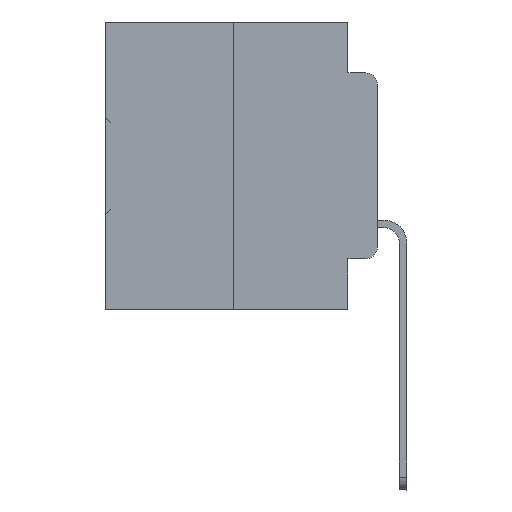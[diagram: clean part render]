
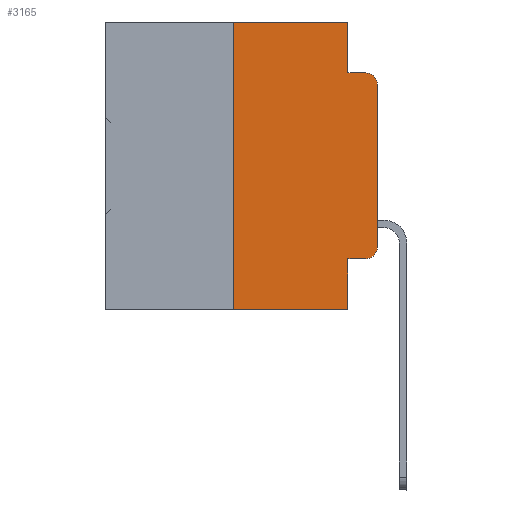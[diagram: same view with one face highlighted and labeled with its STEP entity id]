
A CAD part, left-side view. The second image highlights one B-rep face of the part: STEP entity #3165.
In plain terms, the highlighted planar face has unit normal (-1, 0, 0).
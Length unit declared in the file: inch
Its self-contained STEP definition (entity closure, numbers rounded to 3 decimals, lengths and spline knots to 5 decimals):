
#842 = VERTEX_POINT ( 'NONE', #8794 ) ;
#2227 = CARTESIAN_POINT ( 'NONE',  ( 0., 0.473, 0. ) ) ;
#2470 = EDGE_CURVE ( 'NONE', #12422, #8862, #34350, .T. ) ;
#3095 = DIRECTION ( 'NONE',  ( 0., 0., -1. ) ) ;
#3165 = ADVANCED_FACE ( 'NONE', ( #5425 ), #16175, .F. ) ;
#3203 = EDGE_CURVE ( 'NONE', #30793, #17209, #19401, .T. ) ;
#3281 = DIRECTION ( 'NONE',  ( 0., -1., 0. ) ) ;
#3731 = DIRECTION ( 'NONE',  ( 0., 0., 1. ) ) ;
#3785 = EDGE_CURVE ( 'NONE', #31473, #30793, #11796, .T. ) ;
#5024 = EDGE_CURVE ( 'NONE', #34529, #12422, #36636, .T. ) ;
#5371 = DIRECTION ( 'NONE',  ( 0., -1., 0. ) ) ;
#5425 = FACE_OUTER_BOUND ( 'NONE', #35494, .T. ) ;
#6071 = CARTESIAN_POINT ( 'NONE',  ( 0., 0.051, -0.4115 ) ) ;
#6695 = CARTESIAN_POINT ( 'NONE',  ( 0., 0.02, -0.4115 ) ) ;
#6772 = VERTEX_POINT ( 'NONE', #8458 ) ;
#7511 = DIRECTION ( 'NONE',  ( 0., 0., -1. ) ) ;
#7954 = CARTESIAN_POINT ( 'NONE',  ( 0., 0.051, -0.4115 ) ) ;
#8458 = CARTESIAN_POINT ( 'NONE',  ( 0., 0., -0.1085 ) ) ;
#8794 = CARTESIAN_POINT ( 'NONE',  ( 0., 0.051, -0.0885 ) ) ;
#8862 = VERTEX_POINT ( 'NONE', #14887 ) ;
#9082 = DIRECTION ( 'NONE',  ( -1., 0., 0. ) ) ;
#9260 = LINE ( 'NONE', #12468, #31121 ) ;
#9449 = DIRECTION ( 'NONE',  ( 0., 0., -1. ) ) ;
#11107 = DIRECTION ( 'NONE',  ( 1., 0., 0. ) ) ;
#11164 = VECTOR ( 'NONE', #29727, 39.37008 ) ;
#11585 = CARTESIAN_POINT ( 'NONE',  ( 0., 0.473, -0.5 ) ) ;
#11796 = LINE ( 'NONE', #25756, #29286 ) ;
#12168 = VECTOR ( 'NONE', #5371, 39.37008 ) ;
#12422 = VERTEX_POINT ( 'NONE', #6695 ) ;
#12468 = CARTESIAN_POINT ( 'NONE',  ( 0., 0.051, 0. ) ) ;
#12477 = DIRECTION ( 'NONE',  ( 0., 0., -1. ) ) ;
#12988 = ORIENTED_EDGE ( 'NONE', *, *, #3203, .F. ) ;
#13406 = ORIENTED_EDGE ( 'NONE', *, *, #15177, .T. ) ;
#14860 = LINE ( 'NONE', #18077, #25777 ) ;
#14887 = CARTESIAN_POINT ( 'NONE',  ( 0., 0., -0.3915 ) ) ;
#15177 = EDGE_CURVE ( 'NONE', #8862, #6772, #14860, .T. ) ;
#15397 = EDGE_CURVE ( 'NONE', #31473, #36614, #35158, .T. ) ;
#15567 = CARTESIAN_POINT ( 'NONE',  ( 0., 0.051, -0.5 ) ) ;
#15919 = CARTESIAN_POINT ( 'NONE',  ( 0., 0.25, -0.5 ) ) ;
#15956 = ORIENTED_EDGE ( 'NONE', *, *, #2470, .T. ) ;
#16175 = PLANE ( 'NONE',  #22201 ) ;
#16415 = ORIENTED_EDGE ( 'NONE', *, *, #15397, .T. ) ;
#17209 = VERTEX_POINT ( 'NONE', #24114 ) ;
#18077 = CARTESIAN_POINT ( 'NONE',  ( 0., 0., 0. ) ) ;
#19140 = EDGE_CURVE ( 'NONE', #842, #36525, #20076, .T. ) ;
#19401 = LINE ( 'NONE', #2227, #35459 ) ;
#19473 = DIRECTION ( 'NONE',  ( 0., -1., 0. ) ) ;
#19729 = EDGE_CURVE ( 'NONE', #6772, #36525, #27865, .T. ) ;
#20076 = LINE ( 'NONE', #31231, #12168 ) ;
#20080 = DIRECTION ( 'NONE',  ( -1., 0., 0. ) ) ;
#21246 = EDGE_CURVE ( 'NONE', #17209, #842, #9260, .T. ) ;
#21677 = AXIS2_PLACEMENT_3D ( 'NONE', #28585, #20080, #3095 ) ;
#22201 = AXIS2_PLACEMENT_3D ( 'NONE', #37130, #11107, #7511 ) ;
#22778 = ORIENTED_EDGE ( 'NONE', *, *, #19729, .T. ) ;
#23301 = DIRECTION ( 'NONE',  ( 0., 0., 1. ) ) ;
#23436 = ORIENTED_EDGE ( 'NONE', *, *, #3785, .F. ) ;
#24114 = CARTESIAN_POINT ( 'NONE',  ( 0., 0.051, 0. ) ) ;
#25756 = CARTESIAN_POINT ( 'NONE',  ( 0., 0.25, 0. ) ) ;
#25777 = VECTOR ( 'NONE', #3731, 39.37008 ) ;
#26956 = CARTESIAN_POINT ( 'NONE',  ( 0., 0.25, 0. ) ) ;
#27865 = CIRCLE ( 'NONE', #30884, 0.02 ) ;
#27866 = ORIENTED_EDGE ( 'NONE', *, *, #5024, .T. ) ;
#28348 = ORIENTED_EDGE ( 'NONE', *, *, #37092, .F. ) ;
#28585 = CARTESIAN_POINT ( 'NONE',  ( 0., 0.02, -0.3915 ) ) ;
#29183 = ORIENTED_EDGE ( 'NONE', *, *, #19140, .F. ) ;
#29286 = VECTOR ( 'NONE', #23301, 39.37008 ) ;
#29465 = VECTOR ( 'NONE', #19473, 39.37008 ) ;
#29727 = DIRECTION ( 'NONE',  ( 0., 0., -1. ) ) ;
#30641 = VECTOR ( 'NONE', #3281, 39.37008 ) ;
#30793 = VERTEX_POINT ( 'NONE', #26956 ) ;
#30884 = AXIS2_PLACEMENT_3D ( 'NONE', #34940, #9082, #12477 ) ;
#30924 = DIRECTION ( 'NONE',  ( 0., -1., 0. ) ) ;
#31121 = VECTOR ( 'NONE', #9449, 39.37008 ) ;
#31231 = CARTESIAN_POINT ( 'NONE',  ( 0., 0.051, -0.0885 ) ) ;
#31473 = VERTEX_POINT ( 'NONE', #15919 ) ;
#32186 = LINE ( 'NONE', #35753, #11164 ) ;
#33566 = CARTESIAN_POINT ( 'NONE',  ( 0., 0.02, -0.0885 ) ) ;
#34350 = CIRCLE ( 'NONE', #21677, 0.02 ) ;
#34529 = VERTEX_POINT ( 'NONE', #6071 ) ;
#34940 = CARTESIAN_POINT ( 'NONE',  ( 0., 0.02, -0.1085 ) ) ;
#35158 = LINE ( 'NONE', #11585, #30641 ) ;
#35459 = VECTOR ( 'NONE', #30924, 39.37008 ) ;
#35494 = EDGE_LOOP ( 'NONE', ( #13406, #22778, #29183, #35908, #12988, #23436, #16415, #28348, #27866, #15956 ) ) ;
#35753 = CARTESIAN_POINT ( 'NONE',  ( 0., 0.051, 0. ) ) ;
#35908 = ORIENTED_EDGE ( 'NONE', *, *, #21246, .F. ) ;
#36525 = VERTEX_POINT ( 'NONE', #33566 ) ;
#36614 = VERTEX_POINT ( 'NONE', #15567 ) ;
#36636 = LINE ( 'NONE', #7954, #29465 ) ;
#37092 = EDGE_CURVE ( 'NONE', #34529, #36614, #32186, .T. ) ;
#37130 = CARTESIAN_POINT ( 'NONE',  ( 0., 0.473, 0. ) ) ;
